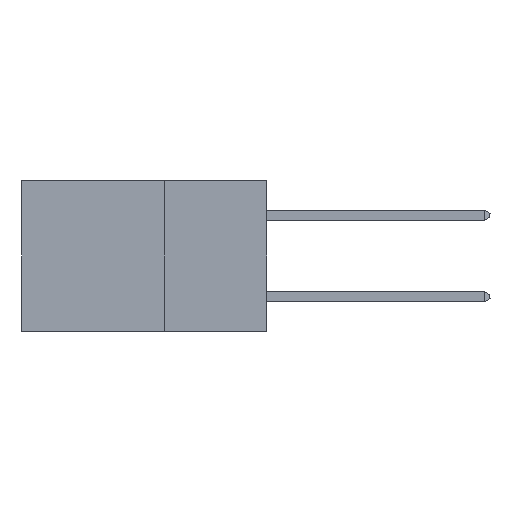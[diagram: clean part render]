
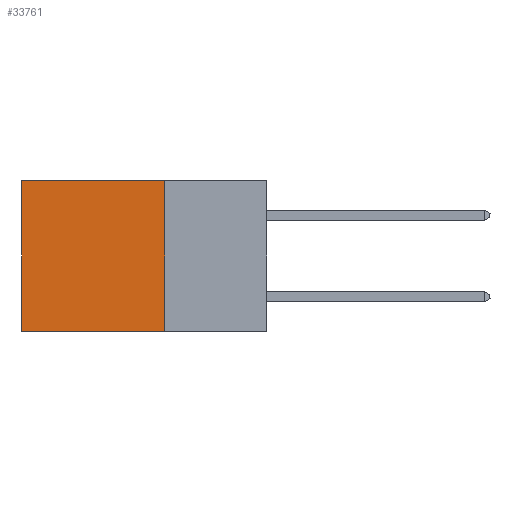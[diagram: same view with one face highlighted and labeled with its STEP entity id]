
A CAD part, left-side view. The second image highlights one B-rep face of the part: STEP entity #33761.
In plain terms, the highlighted planar face has unit normal (-1, 0, 0).
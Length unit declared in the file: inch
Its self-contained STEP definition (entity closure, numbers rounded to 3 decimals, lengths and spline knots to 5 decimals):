
#495 = VECTOR ( 'NONE', #7285, 39.37008 ) ;
#1486 = CARTESIAN_POINT ( 'NONE',  ( 0.2875, 0.6, 0. ) ) ;
#4300 = CARTESIAN_POINT ( 'NONE',  ( 0.2875, 0.25, -0.37 ) ) ;
#4938 = VERTEX_POINT ( 'NONE', #14125 ) ;
#5404 = LINE ( 'NONE', #29803, #35254 ) ;
#6080 = CARTESIAN_POINT ( 'NONE',  ( 0.2875, 0.25, -0.37 ) ) ;
#6927 = FACE_OUTER_BOUND ( 'NONE', #16464, .T. ) ;
#7206 = VERTEX_POINT ( 'NONE', #6080 ) ;
#7261 = EDGE_CURVE ( 'NONE', #4938, #7206, #9171, .T. ) ;
#7285 = DIRECTION ( 'NONE',  ( 0., 1., 0. ) ) ;
#7305 = EDGE_CURVE ( 'NONE', #31520, #31431, #5404, .T. ) ;
#8776 = DIRECTION ( 'NONE',  ( 0., 0., -1. ) ) ;
#8905 = ORIENTED_EDGE ( 'NONE', *, *, #10736, .F. ) ;
#9171 = LINE ( 'NONE', #29672, #29489 ) ;
#9620 = DIRECTION ( 'NONE',  ( 0., 0., -1. ) ) ;
#10736 = EDGE_CURVE ( 'NONE', #7206, #31431, #31448, .T. ) ;
#11473 = ORIENTED_EDGE ( 'NONE', *, *, #7261, .F. ) ;
#13573 = VECTOR ( 'NONE', #34548, 39.37008 ) ;
#14125 = CARTESIAN_POINT ( 'NONE',  ( 0.2875, 0.25, 0. ) ) ;
#14494 = CARTESIAN_POINT ( 'NONE',  ( 0.2875, 0.25, 0. ) ) ;
#16464 = EDGE_LOOP ( 'NONE', ( #24104, #8905, #11473, #20558 ) ) ;
#16545 = EDGE_CURVE ( 'NONE', #4938, #31520, #28013, .T. ) ;
#20558 = ORIENTED_EDGE ( 'NONE', *, *, #16545, .T. ) ;
#24104 = ORIENTED_EDGE ( 'NONE', *, *, #7305, .T. ) ;
#26136 = DIRECTION ( 'NONE',  ( 1., 0., 0. ) ) ;
#28013 = LINE ( 'NONE', #14494, #13573 ) ;
#29489 = VECTOR ( 'NONE', #32551, 39.37008 ) ;
#29672 = CARTESIAN_POINT ( 'NONE',  ( 0.2875, 0.25, 0. ) ) ;
#29803 = CARTESIAN_POINT ( 'NONE',  ( 0.2875, 0.6, 0. ) ) ;
#31431 = VERTEX_POINT ( 'NONE', #33113 ) ;
#31448 = LINE ( 'NONE', #4300, #495 ) ;
#31520 = VERTEX_POINT ( 'NONE', #1486 ) ;
#31737 = CARTESIAN_POINT ( 'NONE',  ( 0.2875, 0.25, 0. ) ) ;
#32551 = DIRECTION ( 'NONE',  ( 0., 0., -1. ) ) ;
#33113 = CARTESIAN_POINT ( 'NONE',  ( 0.2875, 0.6, -0.37 ) ) ;
#33761 = ADVANCED_FACE ( 'NONE', ( #6927 ), #37416, .F. ) ;
#34548 = DIRECTION ( 'NONE',  ( 0., 1., 0. ) ) ;
#34829 = AXIS2_PLACEMENT_3D ( 'NONE', #31737, #26136, #8776 ) ;
#35254 = VECTOR ( 'NONE', #9620, 39.37008 ) ;
#37416 = PLANE ( 'NONE',  #34829 ) ;
